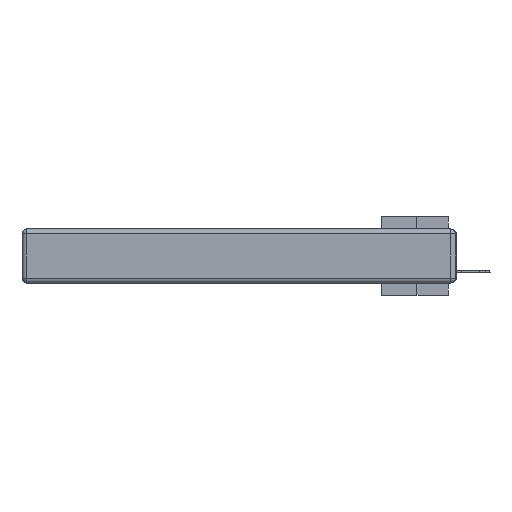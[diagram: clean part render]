
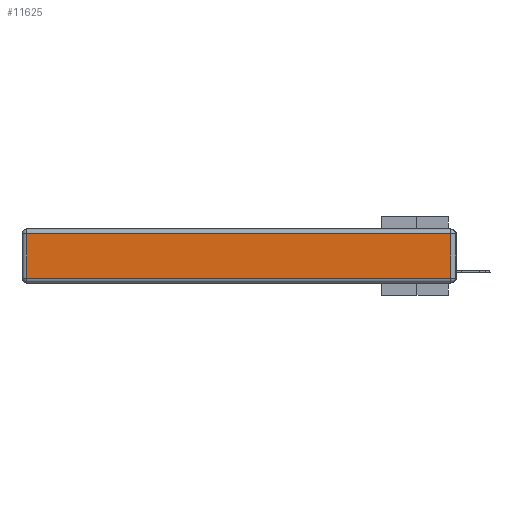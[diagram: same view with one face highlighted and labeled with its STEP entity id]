
A CAD part, left-side view. The second image highlights one B-rep face of the part: STEP entity #11625.
In plain terms, the highlighted planar face has unit normal (-1, 0, 0).
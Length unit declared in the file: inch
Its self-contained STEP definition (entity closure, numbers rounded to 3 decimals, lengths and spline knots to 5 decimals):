
#858 = CARTESIAN_POINT ( 'NONE',  ( 0., 2.72, -0.03 ) ) ;
#1169 = DIRECTION ( 'NONE',  ( 0., -1., 0. ) ) ;
#1560 = ORIENTED_EDGE ( 'NONE', *, *, #22125, .T. ) ;
#1695 = VERTEX_POINT ( 'NONE', #858 ) ;
#2940 = CARTESIAN_POINT ( 'NONE',  ( 0., 0., -0.313 ) ) ;
#6419 = DIRECTION ( 'NONE',  ( 0., 0., 1. ) ) ;
#6612 = DIRECTION ( 'NONE',  ( -1., 0., 0. ) ) ;
#6669 = VERTEX_POINT ( 'NONE', #29069 ) ;
#7784 = VERTEX_POINT ( 'NONE', #28346 ) ;
#8441 = DIRECTION ( 'NONE',  ( 0., 1., 0. ) ) ;
#8977 = DIRECTION ( 'NONE',  ( 0., 0., 1. ) ) ;
#11184 = CARTESIAN_POINT ( 'NONE',  ( 0., 2.72, -0.343 ) ) ;
#11625 = ADVANCED_FACE ( 'NONE', ( #20007 ), #22942, .T. ) ;
#11891 = ORIENTED_EDGE ( 'NONE', *, *, #17270, .T. ) ;
#12821 = CARTESIAN_POINT ( 'NONE',  ( 0., 0.03, -0.343 ) ) ;
#13834 = VECTOR ( 'NONE', #25109, 39.37008 ) ;
#15824 = CARTESIAN_POINT ( 'NONE',  ( 0., 0., -0.343 ) ) ;
#16526 = VECTOR ( 'NONE', #6419, 39.37008 ) ;
#17270 = EDGE_CURVE ( 'NONE', #24206, #7784, #18026, .T. ) ;
#17904 = EDGE_LOOP ( 'NONE', ( #26018, #11891, #1560, #19699 ) ) ;
#18026 = LINE ( 'NONE', #12821, #16526 ) ;
#18709 = EDGE_CURVE ( 'NONE', #1695, #6669, #22316, .T. ) ;
#19309 = EDGE_CURVE ( 'NONE', #6669, #24206, #28147, .T. ) ;
#19699 = ORIENTED_EDGE ( 'NONE', *, *, #18709, .T. ) ;
#20007 = FACE_OUTER_BOUND ( 'NONE', #17904, .T. ) ;
#20604 = AXIS2_PLACEMENT_3D ( 'NONE', #15824, #6612, #8977 ) ;
#21512 = VECTOR ( 'NONE', #8441, 39.37008 ) ;
#22125 = EDGE_CURVE ( 'NONE', #7784, #1695, #28335, .T. ) ;
#22316 = LINE ( 'NONE', #11184, #13834 ) ;
#22942 = PLANE ( 'NONE',  #20604 ) ;
#24206 = VERTEX_POINT ( 'NONE', #25351 ) ;
#25109 = DIRECTION ( 'NONE',  ( 0., 0., -1. ) ) ;
#25351 = CARTESIAN_POINT ( 'NONE',  ( 0., 0.03, -0.313 ) ) ;
#26018 = ORIENTED_EDGE ( 'NONE', *, *, #19309, .T. ) ;
#27570 = VECTOR ( 'NONE', #1169, 39.37008 ) ;
#28147 = LINE ( 'NONE', #2940, #27570 ) ;
#28335 = LINE ( 'NONE', #28763, #21512 ) ;
#28346 = CARTESIAN_POINT ( 'NONE',  ( 0., 0.03, -0.03 ) ) ;
#28763 = CARTESIAN_POINT ( 'NONE',  ( 0., 2.75, -0.03 ) ) ;
#29069 = CARTESIAN_POINT ( 'NONE',  ( 0., 2.72, -0.313 ) ) ;
